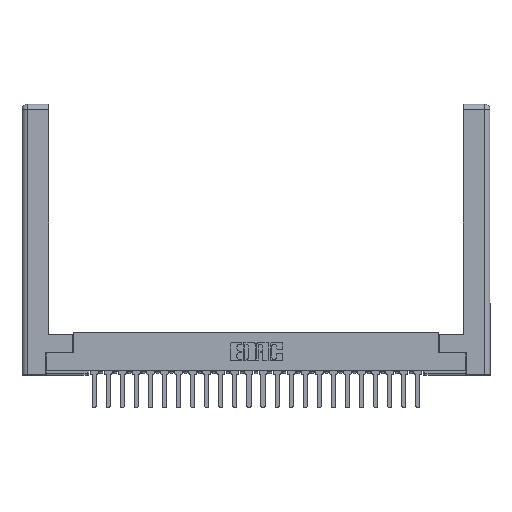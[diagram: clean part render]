
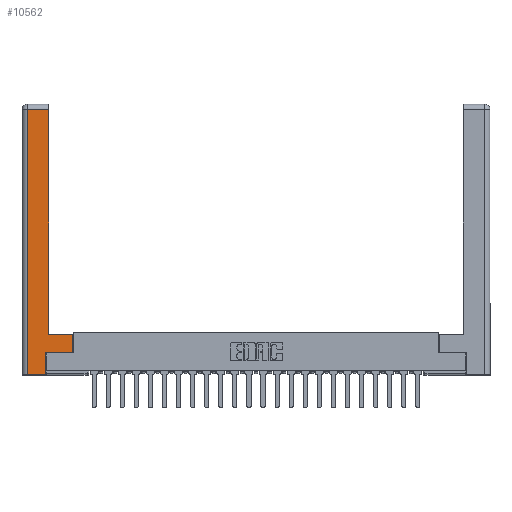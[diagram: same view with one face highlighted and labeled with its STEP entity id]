
A CAD part, top view. The second image highlights one B-rep face of the part: STEP entity #10562.
In plain terms, the highlighted planar face has unit normal (0, 0, 1).
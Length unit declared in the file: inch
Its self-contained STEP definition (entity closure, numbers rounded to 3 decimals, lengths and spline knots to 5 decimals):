
#690 = VERTEX_POINT ( 'NONE', #14642 ) ;
#793 = LINE ( 'NONE', #22135, #12722 ) ;
#824 = DIRECTION ( 'NONE',  ( 0., 1., 0. ) ) ;
#1499 = CARTESIAN_POINT ( 'NONE',  ( 0.565, 0.45, 0. ) ) ;
#1526 = ORIENTED_EDGE ( 'NONE', *, *, #13586, .T. ) ;
#1698 = ORIENTED_EDGE ( 'NONE', *, *, #2845, .T. ) ;
#2228 = VECTOR ( 'NONE', #22504, 39.37008 ) ;
#2845 = EDGE_CURVE ( 'NONE', #6033, #20930, #25398, .T. ) ;
#3239 = CARTESIAN_POINT ( 'NONE',  ( 0.265, 0.245, 0. ) ) ;
#3434 = DIRECTION ( 'NONE',  ( 0., 1., 0. ) ) ;
#4150 = VERTEX_POINT ( 'NONE', #19249 ) ;
#4325 = VECTOR ( 'NONE', #9746, 39.37008 ) ;
#4774 = EDGE_CURVE ( 'NONE', #4150, #19329, #7105, .T. ) ;
#5352 = LINE ( 'NONE', #19100, #9095 ) ;
#5360 = EDGE_CURVE ( 'NONE', #690, #5962, #17094, .T. ) ;
#5690 = VECTOR ( 'NONE', #23049, 39.37008 ) ;
#5962 = VERTEX_POINT ( 'NONE', #3239 ) ;
#6033 = VERTEX_POINT ( 'NONE', #15545 ) ;
#6323 = ORIENTED_EDGE ( 'NONE', *, *, #9283, .T. ) ;
#6547 = CARTESIAN_POINT ( 'NONE',  ( 0., 0., 0. ) ) ;
#7005 = VERTEX_POINT ( 'NONE', #18055 ) ;
#7105 = LINE ( 'NONE', #20347, #2228 ) ;
#7243 = VERTEX_POINT ( 'NONE', #21454 ) ;
#7914 = ORIENTED_EDGE ( 'NONE', *, *, #4774, .T. ) ;
#9065 = CARTESIAN_POINT ( 'NONE',  ( 0.295, 3., 0. ) ) ;
#9076 = CARTESIAN_POINT ( 'NONE',  ( 0.295, 0.45, 0. ) ) ;
#9095 = VECTOR ( 'NONE', #25253, 39.37008 ) ;
#9101 = FACE_OUTER_BOUND ( 'NONE', #19129, .T. ) ;
#9125 = ORIENTED_EDGE ( 'NONE', *, *, #21872, .T. ) ;
#9283 = EDGE_CURVE ( 'NONE', #20930, #7243, #13316, .T. ) ;
#9746 = DIRECTION ( 'NONE',  ( 0., 1., 0. ) ) ;
#10562 = ADVANCED_FACE ( 'NONE', ( #9101 ), #16929, .F. ) ;
#12444 = DIRECTION ( 'NONE',  ( 0., 0., -1. ) ) ;
#12722 = VECTOR ( 'NONE', #18801, 39.37008 ) ;
#12975 = CARTESIAN_POINT ( 'NONE',  ( 0.0615, 2.94, 0. ) ) ;
#13316 = LINE ( 'NONE', #9076, #5690 ) ;
#13586 = EDGE_CURVE ( 'NONE', #7005, #690, #5352, .T. ) ;
#14470 = LINE ( 'NONE', #9065, #18850 ) ;
#14642 = CARTESIAN_POINT ( 'NONE',  ( 0.265, 0., 0. ) ) ;
#15048 = CARTESIAN_POINT ( 'NONE',  ( 0.265, 0.245, 0. ) ) ;
#15510 = ORIENTED_EDGE ( 'NONE', *, *, #18197, .T. ) ;
#15515 = DIRECTION ( 'NONE',  ( -1., 0., 0. ) ) ;
#15545 = CARTESIAN_POINT ( 'NONE',  ( 0.565, 0.245, 0. ) ) ;
#16929 = PLANE ( 'NONE',  #24145 ) ;
#17094 = LINE ( 'NONE', #15048, #4325 ) ;
#17690 = CARTESIAN_POINT ( 'NONE',  ( 0.565, 0.245, 0. ) ) ;
#18055 = CARTESIAN_POINT ( 'NONE',  ( 0.0615, 0., 0. ) ) ;
#18197 = EDGE_CURVE ( 'NONE', #5962, #6033, #19365, .T. ) ;
#18801 = DIRECTION ( 'NONE',  ( 0., -1., 0. ) ) ;
#18850 = VECTOR ( 'NONE', #824, 39.37008 ) ;
#19100 = CARTESIAN_POINT ( 'NONE',  ( 0.265, 0., 0. ) ) ;
#19129 = EDGE_LOOP ( 'NONE', ( #23738, #7914, #9125, #1526, #24495, #15510, #1698, #6323 ) ) ;
#19249 = CARTESIAN_POINT ( 'NONE',  ( 0.295, 2.94, 0. ) ) ;
#19329 = VERTEX_POINT ( 'NONE', #12975 ) ;
#19365 = LINE ( 'NONE', #17690, #22461 ) ;
#20347 = CARTESIAN_POINT ( 'NONE',  ( 0.0615, 2.94, 0. ) ) ;
#20930 = VERTEX_POINT ( 'NONE', #22077 ) ;
#21454 = CARTESIAN_POINT ( 'NONE',  ( 0.295, 0.45, 0. ) ) ;
#21526 = EDGE_CURVE ( 'NONE', #7243, #4150, #14470, .T. ) ;
#21663 = DIRECTION ( 'NONE',  ( 1., 0., 0. ) ) ;
#21872 = EDGE_CURVE ( 'NONE', #19329, #7005, #793, .T. ) ;
#22077 = CARTESIAN_POINT ( 'NONE',  ( 0.565, 0.45, 0. ) ) ;
#22135 = CARTESIAN_POINT ( 'NONE',  ( 0.0615, 0., 0. ) ) ;
#22461 = VECTOR ( 'NONE', #21663, 39.37008 ) ;
#22504 = DIRECTION ( 'NONE',  ( -1., 0., 0. ) ) ;
#23049 = DIRECTION ( 'NONE',  ( -1., 0., 0. ) ) ;
#23738 = ORIENTED_EDGE ( 'NONE', *, *, #21526, .T. ) ;
#24145 = AXIS2_PLACEMENT_3D ( 'NONE', #6547, #12444, #15515 ) ;
#24495 = ORIENTED_EDGE ( 'NONE', *, *, #5360, .T. ) ;
#25024 = VECTOR ( 'NONE', #3434, 39.37008 ) ;
#25253 = DIRECTION ( 'NONE',  ( 1., 0., 0. ) ) ;
#25398 = LINE ( 'NONE', #1499, #25024 ) ;
